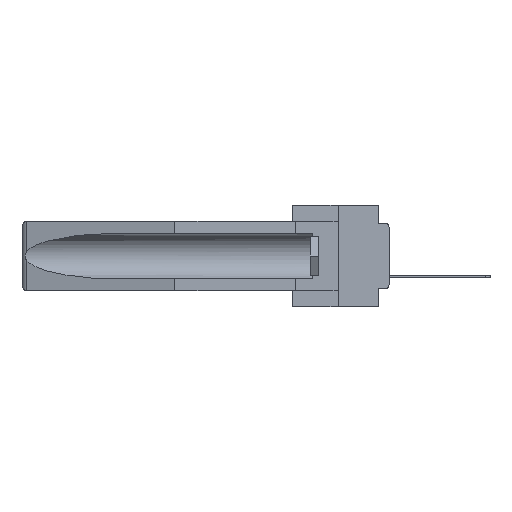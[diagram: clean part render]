
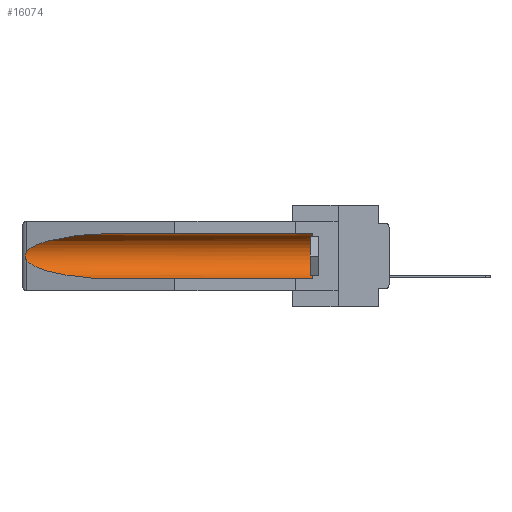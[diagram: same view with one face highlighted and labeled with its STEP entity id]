
A CAD part, left-side view. The second image highlights one B-rep face of the part: STEP entity #16074.
In plain terms, the highlighted cylindrical face has radius 2.857 mm (diameter 5.715 mm), a partial arc.
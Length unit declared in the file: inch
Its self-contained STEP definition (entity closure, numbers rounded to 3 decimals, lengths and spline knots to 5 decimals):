
#94 = CARTESIAN_POINT ( 'NONE',  ( 0.21114, 1.30732, -0.284 ) ) ;
#484 = EDGE_LOOP ( 'NONE', ( #37471, #8665, #16267, #8378, #21363, #5226 ) ) ;
#1670 = DIRECTION ( 'NONE',  ( 0., 1., 0. ) ) ;
#1680 = DIRECTION ( 'NONE',  ( 0., 0., 1. ) ) ;
#4017 = CARTESIAN_POINT ( 'NONE',  ( 0.2673, 1.5327, -0.16383 ) ) ;
#4371 = DIRECTION ( 'NONE',  ( 0., 1., 0. ) ) ;
#4411 = VERTEX_POINT ( 'NONE', #22002 ) ;
#4804 = FACE_OUTER_BOUND ( 'NONE', #484, .T. ) ;
#4899 = VERTEX_POINT ( 'NONE', #14299 ) ;
#5183 = CYLINDRICAL_SURFACE ( 'NONE', #33043, 0.1125 ) ;
#5226 = ORIENTED_EDGE ( 'NONE', *, *, #31066, .T. ) ;
#6152 = CARTESIAN_POINT ( 'NONE',  ( 0.2675, 1.53308, -0.17534 ) ) ;
#6668 = VERTEX_POINT ( 'NONE', #32060 ) ;
#8378 = ORIENTED_EDGE ( 'NONE', *, *, #17784, .F. ) ;
#8482 = VERTEX_POINT ( 'NONE', #33381 ) ;
#8665 = ORIENTED_EDGE ( 'NONE', *, *, #36089, .T. ) ;
#8902 = EDGE_CURVE ( 'NONE', #8482, #4899, #25133, .T. ) ;
#9075 = CARTESIAN_POINT ( 'NONE',  ( 0.26655, 1.53094, -0.18657 ) ) ;
#11582 = VERTEX_POINT ( 'NONE', #14648 ) ;
#12008 = CARTESIAN_POINT ( 'NONE',  ( 0.26597, 1.5296, -0.19026 ) ) ;
#12516 = CARTESIAN_POINT ( 'NONE',  ( 0.26537, 1.52718, -0.14972 ) ) ;
#14246 = CARTESIAN_POINT ( 'NONE',  ( 0.155, 0.126, -0.059 ) ) ;
#14299 = CARTESIAN_POINT ( 'NONE',  ( 0.26537, 1.52718, -0.14972 ) ) ;
#14648 = CARTESIAN_POINT ( 'NONE',  ( 0.155, 1.07973, -0.284 ) ) ;
#15539 = VECTOR ( 'NONE', #1670, 39.37008 ) ;
#15659 = LINE ( 'NONE', #25193, #15539 ) ;
#15828 = CIRCLE ( 'NONE', #37584, 0.1125 ) ;
#15864 = CARTESIAN_POINT ( 'NONE',  ( 0.2673, 1.53269, -0.17917 ) ) ;
#16074 = ADVANCED_FACE ( 'NONE', ( #4804 ), #5183, .F. ) ;
#16267 = ORIENTED_EDGE ( 'NONE', *, *, #34625, .T. ) ;
#17023 = CARTESIAN_POINT ( 'NONE',  ( 0.155, 0.126, -0.1715 ) ) ;
#17038 = CARTESIAN_POINT ( 'NONE',  ( 0.155, -0.30754, -0.1715 ) ) ;
#17242 = B_SPLINE_CURVE_WITH_KNOTS ( 'NONE', 3,
 ( #30074, #24634, #33585, #4017, #35725, #6152, #15864, #9075, #12008, #20930 ),
 .UNSPECIFIED., .F., .F.,
 ( 4, 2, 2, 2, 4 ),
 ( 0., 0.00029, 0.00058, 0.00087, 0.00117 ),
 .UNSPECIFIED. ) ;
#17784 = EDGE_CURVE ( 'NONE', #4411, #11582, #37444, .T. ) ;
#19139 = CARTESIAN_POINT ( 'NONE',  ( 0.155, -0.30754, -0.284 ) ) ;
#20930 = CARTESIAN_POINT ( 'NONE',  ( 0.26537, 1.52718, -0.19328 ) ) ;
#21363 = ORIENTED_EDGE ( 'NONE', *, *, #24509, .T. ) ;
#22002 = CARTESIAN_POINT ( 'NONE',  ( 0.155, 0.126, -0.284 ) ) ;
#24509 = EDGE_CURVE ( 'NONE', #4411, #32965, #15828, .T. ) ;
#24634 = CARTESIAN_POINT ( 'NONE',  ( 0.26597, 1.52961, -0.15275 ) ) ;
#25029 = DIRECTION ( 'NONE',  ( 0., 0., 1. ) ) ;
#25133 =( BOUNDED_CURVE ( )  B_SPLINE_CURVE ( 3, ( #33527, #33330, #35666, #12516 ),
 .UNSPECIFIED., .F., .T. ) 
 B_SPLINE_CURVE_WITH_KNOTS ( ( 4, 4 ),
 ( 4.71239, 6.08839 ),
 .UNSPECIFIED. ) 
 CURVE ( )  GEOMETRIC_REPRESENTATION_ITEM ( )  RATIONAL_B_SPLINE_CURVE ( ( 1., 0.848, 0.848, 1. ) ) 
 REPRESENTATION_ITEM ( '' )  );
#25193 = CARTESIAN_POINT ( 'NONE',  ( 0.155, -0.30754, -0.059 ) ) ;
#28908 = DIRECTION ( 'NONE',  ( 0., 1., 0. ) ) ;
#29818 = CARTESIAN_POINT ( 'NONE',  ( 0.25451, 1.48313, -0.24835 ) ) ;
#30074 = CARTESIAN_POINT ( 'NONE',  ( 0.26537, 1.52718, -0.14972 ) ) ;
#30808 =( BOUNDED_CURVE ( )  B_SPLINE_CURVE ( 3, ( #32026, #29818, #94, #31837 ),
 .UNSPECIFIED., .F., .T. ) 
 B_SPLINE_CURVE_WITH_KNOTS ( ( 4, 4 ),
 ( 0.1948, 1.5708 ),
 .UNSPECIFIED. ) 
 CURVE ( )  GEOMETRIC_REPRESENTATION_ITEM ( )  RATIONAL_B_SPLINE_CURVE ( ( 1., 0.848, 0.848, 1. ) ) 
 REPRESENTATION_ITEM ( '' )  );
#31066 = EDGE_CURVE ( 'NONE', #32965, #8482, #15659, .T. ) ;
#31837 = CARTESIAN_POINT ( 'NONE',  ( 0.155, 1.07973, -0.284 ) ) ;
#32026 = CARTESIAN_POINT ( 'NONE',  ( 0.26537, 1.52718, -0.19328 ) ) ;
#32060 = CARTESIAN_POINT ( 'NONE',  ( 0.26537, 1.52718, -0.19328 ) ) ;
#32965 = VERTEX_POINT ( 'NONE', #14246 ) ;
#33043 = AXIS2_PLACEMENT_3D ( 'NONE', #17038, #28908, #25029 ) ;
#33330 = CARTESIAN_POINT ( 'NONE',  ( 0.21114, 1.30732, -0.059 ) ) ;
#33381 = CARTESIAN_POINT ( 'NONE',  ( 0.155, 1.07973, -0.059 ) ) ;
#33527 = CARTESIAN_POINT ( 'NONE',  ( 0.155, 1.07973, -0.059 ) ) ;
#33585 = CARTESIAN_POINT ( 'NONE',  ( 0.26654, 1.53092, -0.15636 ) ) ;
#34546 = DIRECTION ( 'NONE',  ( 0., -1., 0. ) ) ;
#34625 = EDGE_CURVE ( 'NONE', #6668, #11582, #30808, .T. ) ;
#35666 = CARTESIAN_POINT ( 'NONE',  ( 0.25451, 1.48313, -0.09465 ) ) ;
#35725 = CARTESIAN_POINT ( 'NONE',  ( 0.2675, 1.53308, -0.16763 ) ) ;
#36089 = EDGE_CURVE ( 'NONE', #4899, #6668, #17242, .T. ) ;
#37386 = VECTOR ( 'NONE', #4371, 39.37008 ) ;
#37444 = LINE ( 'NONE', #19139, #37386 ) ;
#37471 = ORIENTED_EDGE ( 'NONE', *, *, #8902, .T. ) ;
#37584 = AXIS2_PLACEMENT_3D ( 'NONE', #17023, #34546, #1680 ) ;
